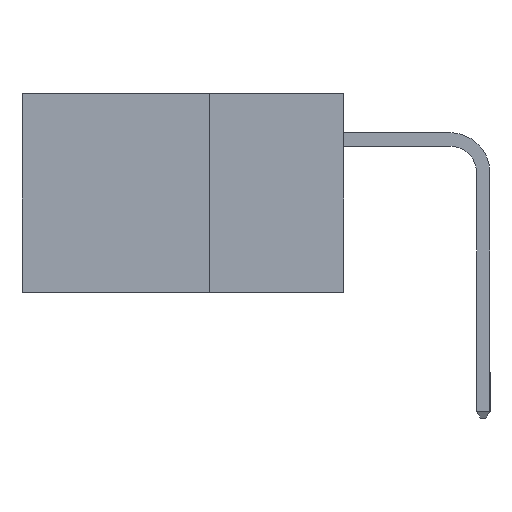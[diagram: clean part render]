
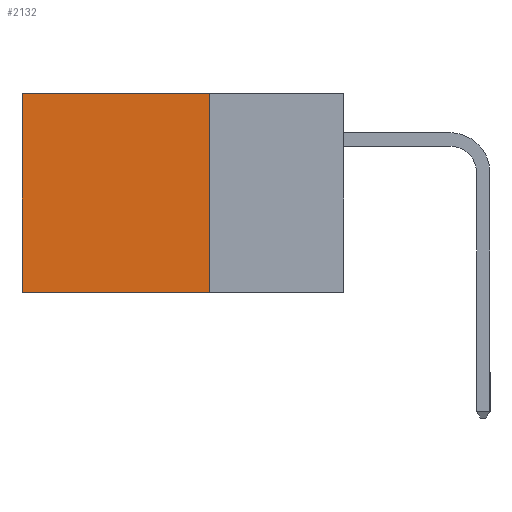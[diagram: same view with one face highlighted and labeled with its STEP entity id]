
A CAD part, left-side view. The second image highlights one B-rep face of the part: STEP entity #2132.
In plain terms, the highlighted planar face has unit normal (-1, 0, 0).
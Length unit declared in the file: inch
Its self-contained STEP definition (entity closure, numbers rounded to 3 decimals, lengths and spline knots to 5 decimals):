
#623 = LINE ( 'NONE', #5055, #16829 ) ;
#928 = EDGE_CURVE ( 'NONE', #5625, #8876, #15528, .T. ) ;
#1124 = ORIENTED_EDGE ( 'NONE', *, *, #5938, .F. ) ;
#1172 = ORIENTED_EDGE ( 'NONE', *, *, #17491, .T. ) ;
#1363 = FACE_OUTER_BOUND ( 'NONE', #17991, .T. ) ;
#1956 = CARTESIAN_POINT ( 'NONE',  ( 0.2615, 0.25, 0. ) ) ;
#2132 = ADVANCED_FACE ( 'NONE', ( #1363 ), #14951, .F. ) ;
#2346 = DIRECTION ( 'NONE',  ( 0., 1., 0. ) ) ;
#5055 = CARTESIAN_POINT ( 'NONE',  ( 0.2615, 0.25, -0.37 ) ) ;
#5157 = VERTEX_POINT ( 'NONE', #8739 ) ;
#5625 = VERTEX_POINT ( 'NONE', #10916 ) ;
#5739 = ORIENTED_EDGE ( 'NONE', *, *, #13621, .F. ) ;
#5938 = EDGE_CURVE ( 'NONE', #17293, #8876, #18049, .T. ) ;
#6672 = LINE ( 'NONE', #1956, #18448 ) ;
#6972 = CARTESIAN_POINT ( 'NONE',  ( 0.2615, 0.6, -0.37 ) ) ;
#8739 = CARTESIAN_POINT ( 'NONE',  ( 0.2615, 0.25, 0. ) ) ;
#8876 = VERTEX_POINT ( 'NONE', #6972 ) ;
#9049 = VECTOR ( 'NONE', #10330, 39.37008 ) ;
#10330 = DIRECTION ( 'NONE',  ( 0., 1., 0. ) ) ;
#10916 = CARTESIAN_POINT ( 'NONE',  ( 0.2615, 0.6, 0. ) ) ;
#11071 = DIRECTION ( 'NONE',  ( 0., 0., -1. ) ) ;
#11335 = VECTOR ( 'NONE', #12566, 39.37008 ) ;
#11909 = DIRECTION ( 'NONE',  ( 0., 0., -1. ) ) ;
#12026 = CARTESIAN_POINT ( 'NONE',  ( 0.2615, 0.25, -0.37 ) ) ;
#12566 = DIRECTION ( 'NONE',  ( 0., 0., -1. ) ) ;
#13621 = EDGE_CURVE ( 'NONE', #5157, #17293, #623, .T. ) ;
#13954 = ORIENTED_EDGE ( 'NONE', *, *, #928, .T. ) ;
#14132 = CARTESIAN_POINT ( 'NONE',  ( 0.2615, 0.6, -0.37 ) ) ;
#14681 = CARTESIAN_POINT ( 'NONE',  ( 0.2615, 0.25, -0.37 ) ) ;
#14951 = PLANE ( 'NONE',  #15249 ) ;
#15249 = AXIS2_PLACEMENT_3D ( 'NONE', #17733, #15969, #11909 ) ;
#15528 = LINE ( 'NONE', #14132, #11335 ) ;
#15969 = DIRECTION ( 'NONE',  ( 1., 0., 0. ) ) ;
#16829 = VECTOR ( 'NONE', #11071, 39.37008 ) ;
#17293 = VERTEX_POINT ( 'NONE', #12026 ) ;
#17491 = EDGE_CURVE ( 'NONE', #5157, #5625, #6672, .T. ) ;
#17733 = CARTESIAN_POINT ( 'NONE',  ( 0.2615, 0.25, -0.37 ) ) ;
#17991 = EDGE_LOOP ( 'NONE', ( #13954, #1124, #5739, #1172 ) ) ;
#18049 = LINE ( 'NONE', #14681, #9049 ) ;
#18448 = VECTOR ( 'NONE', #2346, 39.37008 ) ;
